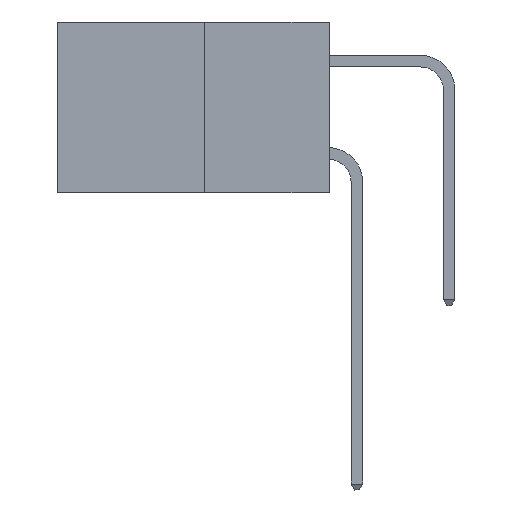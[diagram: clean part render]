
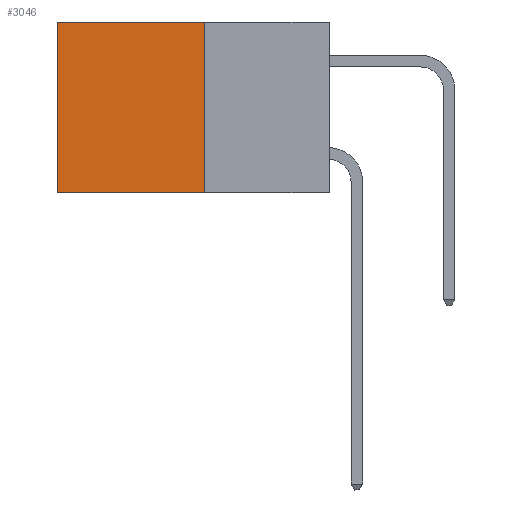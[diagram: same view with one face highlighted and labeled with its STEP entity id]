
A CAD part, left-side view. The second image highlights one B-rep face of the part: STEP entity #3046.
In plain terms, the highlighted planar face has unit normal (-1, 0, 0).
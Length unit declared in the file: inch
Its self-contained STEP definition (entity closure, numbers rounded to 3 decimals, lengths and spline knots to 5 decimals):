
#1261 = LINE ( 'NONE', #19694, #6783 ) ;
#3046 = ADVANCED_FACE ( 'NONE', ( #13269 ), #24408, .F. ) ;
#3177 = CARTESIAN_POINT ( 'NONE',  ( 0.277, 0.27, -0.37 ) ) ;
#3493 = DIRECTION ( 'NONE',  ( 0., 1., 0. ) ) ;
#3804 = CARTESIAN_POINT ( 'NONE',  ( 0.277, 0.27, 0. ) ) ;
#3842 = VECTOR ( 'NONE', #10358, 39.37008 ) ;
#4000 = VERTEX_POINT ( 'NONE', #3804 ) ;
#4265 = VERTEX_POINT ( 'NONE', #21142 ) ;
#5071 = ORIENTED_EDGE ( 'NONE', *, *, #6216, .F. ) ;
#5133 = ORIENTED_EDGE ( 'NONE', *, *, #20248, .F. ) ;
#5390 = EDGE_CURVE ( 'NONE', #4000, #17979, #1261, .T. ) ;
#5946 = LINE ( 'NONE', #11056, #25983 ) ;
#6216 = EDGE_CURVE ( 'NONE', #18973, #4265, #9970, .T. ) ;
#6783 = VECTOR ( 'NONE', #3493, 39.37008 ) ;
#9970 = LINE ( 'NONE', #3177, #3842 ) ;
#10310 = AXIS2_PLACEMENT_3D ( 'NONE', #25065, #15707, #15789 ) ;
#10358 = DIRECTION ( 'NONE',  ( 0., 1., 0. ) ) ;
#10572 = EDGE_LOOP ( 'NONE', ( #14696, #5071, #5133, #20581 ) ) ;
#11056 = CARTESIAN_POINT ( 'NONE',  ( 0.277, 0.27, -0.37 ) ) ;
#11391 = CARTESIAN_POINT ( 'NONE',  ( 0.277, 0.27, -0.37 ) ) ;
#13269 = FACE_OUTER_BOUND ( 'NONE', #10572, .T. ) ;
#13674 = CARTESIAN_POINT ( 'NONE',  ( 0.277, 0.59, 0. ) ) ;
#14518 = LINE ( 'NONE', #23447, #24339 ) ;
#14696 = ORIENTED_EDGE ( 'NONE', *, *, #25727, .T. ) ;
#15707 = DIRECTION ( 'NONE',  ( 1., 0., 0. ) ) ;
#15789 = DIRECTION ( 'NONE',  ( 0., 0., -1. ) ) ;
#17979 = VERTEX_POINT ( 'NONE', #13674 ) ;
#18973 = VERTEX_POINT ( 'NONE', #11391 ) ;
#19694 = CARTESIAN_POINT ( 'NONE',  ( 0.277, 0.27, 0. ) ) ;
#20248 = EDGE_CURVE ( 'NONE', #4000, #18973, #5946, .T. ) ;
#20581 = ORIENTED_EDGE ( 'NONE', *, *, #5390, .T. ) ;
#21142 = CARTESIAN_POINT ( 'NONE',  ( 0.277, 0.59, -0.37 ) ) ;
#23447 = CARTESIAN_POINT ( 'NONE',  ( 0.277, 0.59, -0.37 ) ) ;
#24339 = VECTOR ( 'NONE', #25478, 39.37008 ) ;
#24408 = PLANE ( 'NONE',  #10310 ) ;
#24922 = DIRECTION ( 'NONE',  ( 0., 0., -1. ) ) ;
#25065 = CARTESIAN_POINT ( 'NONE',  ( 0.277, 0.27, -0.37 ) ) ;
#25478 = DIRECTION ( 'NONE',  ( 0., 0., -1. ) ) ;
#25727 = EDGE_CURVE ( 'NONE', #17979, #4265, #14518, .T. ) ;
#25983 = VECTOR ( 'NONE', #24922, 39.37008 ) ;
